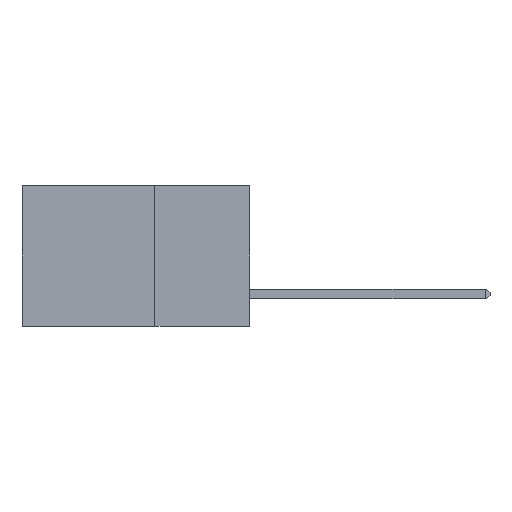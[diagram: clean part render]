
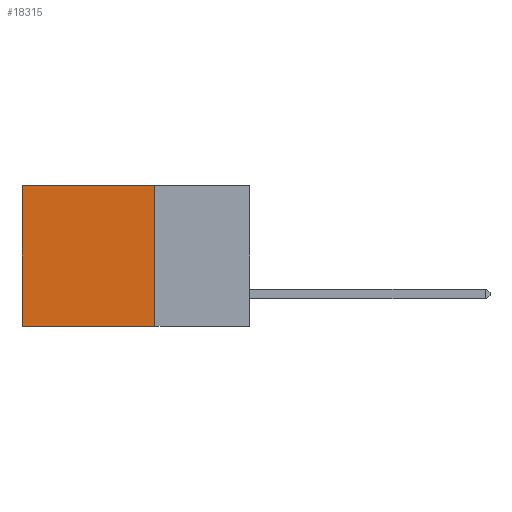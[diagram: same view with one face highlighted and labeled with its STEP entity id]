
A CAD part, left-side view. The second image highlights one B-rep face of the part: STEP entity #18315.
In plain terms, the highlighted planar face has unit normal (-1, 0, 0).
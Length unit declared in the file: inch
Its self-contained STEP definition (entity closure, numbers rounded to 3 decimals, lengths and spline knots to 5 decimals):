
#284 = VERTEX_POINT ( 'NONE', #12381 ) ;
#744 = CARTESIAN_POINT ( 'NONE',  ( 0.2875, 0.6, -0.37 ) ) ;
#1436 = DIRECTION ( 'NONE',  ( 0., 1., 0. ) ) ;
#1499 = ORIENTED_EDGE ( 'NONE', *, *, #9241, .T. ) ;
#1618 = PLANE ( 'NONE',  #14933 ) ;
#4254 = VERTEX_POINT ( 'NONE', #744 ) ;
#4839 = CARTESIAN_POINT ( 'NONE',  ( 0.2875, 0.25, 0. ) ) ;
#5297 = FACE_OUTER_BOUND ( 'NONE', #8387, .T. ) ;
#5492 = DIRECTION ( 'NONE',  ( 1., 0., 0. ) ) ;
#5502 = VECTOR ( 'NONE', #22333, 39.37008 ) ;
#6309 = EDGE_CURVE ( 'NONE', #9461, #284, #18225, .T. ) ;
#6998 = CARTESIAN_POINT ( 'NONE',  ( 0.2875, 0.25, -0.37 ) ) ;
#7281 = CARTESIAN_POINT ( 'NONE',  ( 0.2875, 0.6, 0. ) ) ;
#7707 = ORIENTED_EDGE ( 'NONE', *, *, #7973, .F. ) ;
#7973 = EDGE_CURVE ( 'NONE', #13475, #4254, #20826, .T. ) ;
#8387 = EDGE_LOOP ( 'NONE', ( #1499, #7707, #15655, #12169 ) ) ;
#8622 = VECTOR ( 'NONE', #1436, 39.37008 ) ;
#9241 = EDGE_CURVE ( 'NONE', #284, #4254, #10539, .T. ) ;
#9461 = VERTEX_POINT ( 'NONE', #23148 ) ;
#9930 = VECTOR ( 'NONE', #24455, 39.37008 ) ;
#10527 = DIRECTION ( 'NONE',  ( 0., 0., -1. ) ) ;
#10539 = LINE ( 'NONE', #7281, #9930 ) ;
#12169 = ORIENTED_EDGE ( 'NONE', *, *, #6309, .T. ) ;
#12193 = VECTOR ( 'NONE', #10527, 39.37008 ) ;
#12356 = EDGE_CURVE ( 'NONE', #9461, #13475, #17314, .T. ) ;
#12381 = CARTESIAN_POINT ( 'NONE',  ( 0.2875, 0.6, 0. ) ) ;
#13475 = VERTEX_POINT ( 'NONE', #23236 ) ;
#14933 = AXIS2_PLACEMENT_3D ( 'NONE', #20783, #5492, #18927 ) ;
#15655 = ORIENTED_EDGE ( 'NONE', *, *, #12356, .F. ) ;
#17314 = LINE ( 'NONE', #4839, #12193 ) ;
#18225 = LINE ( 'NONE', #18653, #8622 ) ;
#18315 = ADVANCED_FACE ( 'NONE', ( #5297 ), #1618, .F. ) ;
#18653 = CARTESIAN_POINT ( 'NONE',  ( 0.2875, 0.25, 0. ) ) ;
#18927 = DIRECTION ( 'NONE',  ( 0., 0., -1. ) ) ;
#20783 = CARTESIAN_POINT ( 'NONE',  ( 0.2875, 0.25, 0. ) ) ;
#20826 = LINE ( 'NONE', #6998, #5502 ) ;
#22333 = DIRECTION ( 'NONE',  ( 0., 1., 0. ) ) ;
#23148 = CARTESIAN_POINT ( 'NONE',  ( 0.2875, 0.25, 0. ) ) ;
#23236 = CARTESIAN_POINT ( 'NONE',  ( 0.2875, 0.25, -0.37 ) ) ;
#24455 = DIRECTION ( 'NONE',  ( 0., 0., -1. ) ) ;
